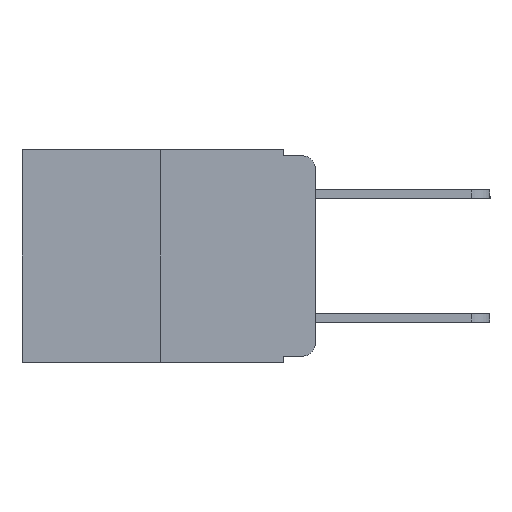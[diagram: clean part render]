
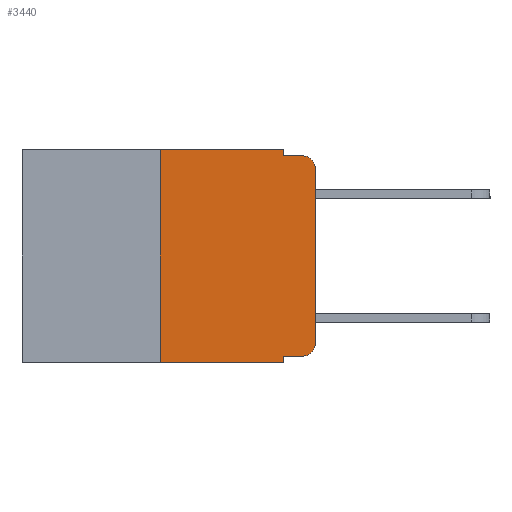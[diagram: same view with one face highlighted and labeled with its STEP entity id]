
A CAD part, left-side view. The second image highlights one B-rep face of the part: STEP entity #3440.
In plain terms, the highlighted planar face has unit normal (-1, 0, 0).
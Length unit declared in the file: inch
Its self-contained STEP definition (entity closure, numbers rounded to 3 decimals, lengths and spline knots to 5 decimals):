
#106 = VERTEX_POINT ( 'NONE', #314 ) ;
#199 = CARTESIAN_POINT ( 'NONE',  ( 0., 0.051, -0.343 ) ) ;
#203 = ORIENTED_EDGE ( 'NONE', *, *, #3042, .F. ) ;
#231 = CARTESIAN_POINT ( 'NONE',  ( 0., 0.02, -0.333 ) ) ;
#272 = LINE ( 'NONE', #6266, #8011 ) ;
#314 = CARTESIAN_POINT ( 'NONE',  ( 0., 0.051, -0.01 ) ) ;
#415 = VECTOR ( 'NONE', #4149, 39.37008 ) ;
#456 = ORIENTED_EDGE ( 'NONE', *, *, #8516, .F. ) ;
#637 = CARTESIAN_POINT ( 'NONE',  ( 0., 0.25, 0. ) ) ;
#653 = LINE ( 'NONE', #4075, #415 ) ;
#798 = ORIENTED_EDGE ( 'NONE', *, *, #4007, .F. ) ;
#1148 = VECTOR ( 'NONE', #7239, 39.37008 ) ;
#1199 = ORIENTED_EDGE ( 'NONE', *, *, #5825, .T. ) ;
#1464 = ORIENTED_EDGE ( 'NONE', *, *, #3691, .F. ) ;
#1655 = ORIENTED_EDGE ( 'NONE', *, *, #6045, .T. ) ;
#1702 = ORIENTED_EDGE ( 'NONE', *, *, #7661, .T. ) ;
#1864 = VERTEX_POINT ( 'NONE', #6086 ) ;
#1900 = CARTESIAN_POINT ( 'NONE',  ( 0., 0.473, 0. ) ) ;
#2036 = VERTEX_POINT ( 'NONE', #5166 ) ;
#2284 = LINE ( 'NONE', #637, #5934 ) ;
#2516 = CARTESIAN_POINT ( 'NONE',  ( 0., 0.02, -0.01 ) ) ;
#2587 = EDGE_CURVE ( 'NONE', #3703, #4177, #8926, .T. ) ;
#2644 = VECTOR ( 'NONE', #6422, 39.37008 ) ;
#2939 = LINE ( 'NONE', #6784, #2644 ) ;
#2945 = VECTOR ( 'NONE', #4899, 39.37008 ) ;
#2993 = DIRECTION ( 'NONE',  ( 0., 0., 1. ) ) ;
#3042 = EDGE_CURVE ( 'NONE', #7273, #106, #653, .T. ) ;
#3155 = CARTESIAN_POINT ( 'NONE',  ( 0., 0.473, 0. ) ) ;
#3223 = VERTEX_POINT ( 'NONE', #199 ) ;
#3236 = LINE ( 'NONE', #3332, #2945 ) ;
#3248 = PLANE ( 'NONE',  #9341 ) ;
#3332 = CARTESIAN_POINT ( 'NONE',  ( 0., 0., 0. ) ) ;
#3351 = EDGE_CURVE ( 'NONE', #106, #4177, #8912, .T. ) ;
#3434 = DIRECTION ( 'NONE',  ( 0., 0., -1. ) ) ;
#3440 = ADVANCED_FACE ( 'NONE', ( #8501 ), #3248, .F. ) ;
#3465 = CARTESIAN_POINT ( 'NONE',  ( 0., 0., -0.313 ) ) ;
#3580 = DIRECTION ( 'NONE',  ( 0., -1., 0. ) ) ;
#3691 = EDGE_CURVE ( 'NONE', #1864, #3223, #272, .T. ) ;
#3703 = VERTEX_POINT ( 'NONE', #6326 ) ;
#3798 = CARTESIAN_POINT ( 'NONE',  ( 0., 0.051, -0.333 ) ) ;
#4007 = EDGE_CURVE ( 'NONE', #2036, #9066, #2284, .T. ) ;
#4075 = CARTESIAN_POINT ( 'NONE',  ( 0., 0.051, 0. ) ) ;
#4149 = DIRECTION ( 'NONE',  ( 0., 0., -1. ) ) ;
#4177 = VERTEX_POINT ( 'NONE', #2516 ) ;
#4184 = VERTEX_POINT ( 'NONE', #3465 ) ;
#4633 = VECTOR ( 'NONE', #3580, 39.37008 ) ;
#4637 = EDGE_CURVE ( 'NONE', #4184, #3703, #3236, .T. ) ;
#4699 = DIRECTION ( 'NONE',  ( 1., 0., 0. ) ) ;
#4899 = DIRECTION ( 'NONE',  ( 0., 0., 1. ) ) ;
#5120 = DIRECTION ( 'NONE',  ( 0., -1., 0. ) ) ;
#5166 = CARTESIAN_POINT ( 'NONE',  ( 0., 0.25, -0.343 ) ) ;
#5184 = AXIS2_PLACEMENT_3D ( 'NONE', #5944, #8834, #5488 ) ;
#5242 = CARTESIAN_POINT ( 'NONE',  ( 0., 0.25, 0. ) ) ;
#5361 = CARTESIAN_POINT ( 'NONE',  ( 0., 0.051, -0.01 ) ) ;
#5396 = VECTOR ( 'NONE', #5120, 39.37008 ) ;
#5488 = DIRECTION ( 'NONE',  ( 0., 0., -1. ) ) ;
#5607 = LINE ( 'NONE', #1900, #1148 ) ;
#5825 = EDGE_CURVE ( 'NONE', #2036, #3223, #2939, .T. ) ;
#5934 = VECTOR ( 'NONE', #2993, 39.37008 ) ;
#5944 = CARTESIAN_POINT ( 'NONE',  ( 0., 0.02, -0.313 ) ) ;
#6045 = EDGE_CURVE ( 'NONE', #1864, #6375, #6496, .T. ) ;
#6086 = CARTESIAN_POINT ( 'NONE',  ( 0., 0.051, -0.333 ) ) ;
#6266 = CARTESIAN_POINT ( 'NONE',  ( 0., 0.051, 0. ) ) ;
#6326 = CARTESIAN_POINT ( 'NONE',  ( 0., 0., -0.03 ) ) ;
#6375 = VERTEX_POINT ( 'NONE', #231 ) ;
#6422 = DIRECTION ( 'NONE',  ( 0., -1., 0. ) ) ;
#6496 = LINE ( 'NONE', #3798, #4633 ) ;
#6522 = DIRECTION ( 'NONE',  ( 0., 0., -1. ) ) ;
#6784 = CARTESIAN_POINT ( 'NONE',  ( 0., 0.473, -0.343 ) ) ;
#6906 = AXIS2_PLACEMENT_3D ( 'NONE', #8789, #8824, #8888 ) ;
#7239 = DIRECTION ( 'NONE',  ( 0., -1., 0. ) ) ;
#7273 = VERTEX_POINT ( 'NONE', #7324 ) ;
#7324 = CARTESIAN_POINT ( 'NONE',  ( 0., 0.051, 0. ) ) ;
#7661 = EDGE_CURVE ( 'NONE', #6375, #4184, #9375, .T. ) ;
#8011 = VECTOR ( 'NONE', #6522, 39.37008 ) ;
#8242 = EDGE_LOOP ( 'NONE', ( #8856, #8956, #9139, #203, #456, #798, #1199, #1464, #1655, #1702 ) ) ;
#8501 = FACE_OUTER_BOUND ( 'NONE', #8242, .T. ) ;
#8516 = EDGE_CURVE ( 'NONE', #9066, #7273, #5607, .T. ) ;
#8789 = CARTESIAN_POINT ( 'NONE',  ( 0., 0.02, -0.03 ) ) ;
#8824 = DIRECTION ( 'NONE',  ( -1., 0., 0. ) ) ;
#8834 = DIRECTION ( 'NONE',  ( -1., 0., 0. ) ) ;
#8856 = ORIENTED_EDGE ( 'NONE', *, *, #4637, .T. ) ;
#8888 = DIRECTION ( 'NONE',  ( 0., 0., -1. ) ) ;
#8912 = LINE ( 'NONE', #5361, #5396 ) ;
#8926 = CIRCLE ( 'NONE', #6906, 0.02 ) ;
#8956 = ORIENTED_EDGE ( 'NONE', *, *, #2587, .T. ) ;
#9066 = VERTEX_POINT ( 'NONE', #5242 ) ;
#9139 = ORIENTED_EDGE ( 'NONE', *, *, #3351, .F. ) ;
#9341 = AXIS2_PLACEMENT_3D ( 'NONE', #3155, #4699, #3434 ) ;
#9375 = CIRCLE ( 'NONE', #5184, 0.02 ) ;
